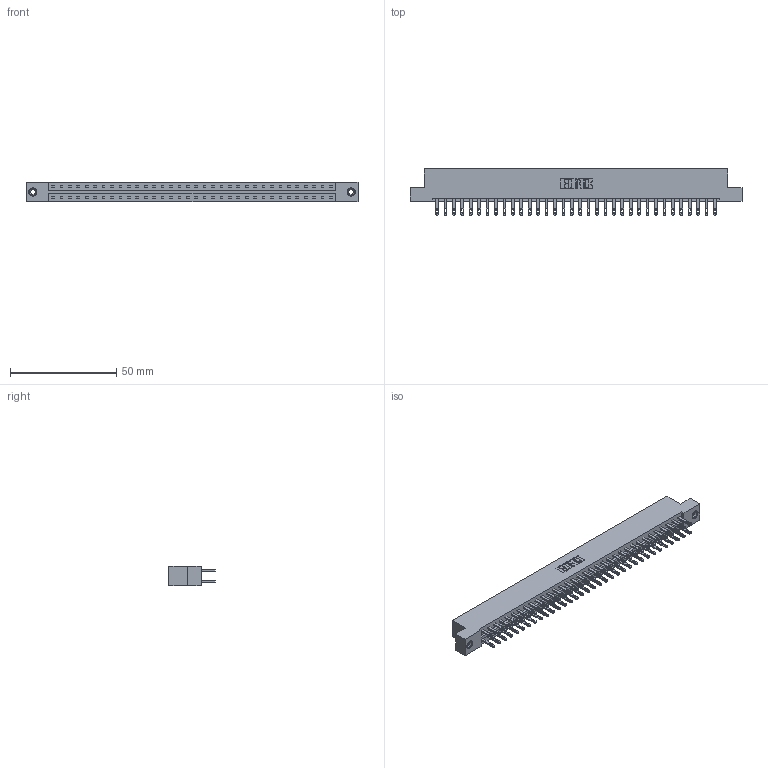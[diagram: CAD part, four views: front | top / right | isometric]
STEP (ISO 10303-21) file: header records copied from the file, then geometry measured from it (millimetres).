
FILE_DESCRIPTION (( 'STEP AP203' ), '1' );
FILE_NAME ('333-068-500-208.STEP', '2018-08-04T12:22:22', ( '' ), ( '' ), 'SwSTEP 2.0', 'SolidWorks 2016', '' );
FILE_SCHEMA (( 'CONFIG_CONTROL_DESIGN' ));
Length unit declared in the file: inch
Products named in the file (4): 333 Part_Flush - .156 Dia - TI; 345-292-001_345-293-100; 345-250-001_345-250-003-102; 333-068-500-208
Assembly tree (71 placements, depth 2):
  333-068-500-208
    333 Part_Flush - .156 Dia - TI
    345-292-001_345-293-100  x68
    345-250-001_345-250-003-102  x2
Bounding box: 156.26 x 21.85 x 9.4 mm (x, y, z)
Volume: 16079.8 mm3; surface area: 19694.4 mm2
Topology: 71 solids, 71 shells, 3438 faces, 10443 edges, 6954 vertices
Faces by surface type: plane 2142, cylinder 1280, cone 12, torus 4
Entity records: 24024 total; most frequent: CARTESIAN_POINT 3973, ORIENTED_EDGE 3902, DIRECTION 3441, EDGE_CURVE 1951, LINE 1799, VECTOR 1799, VERTEX_POINT 1296, AXIS2_PLACEMENT_3D 821
